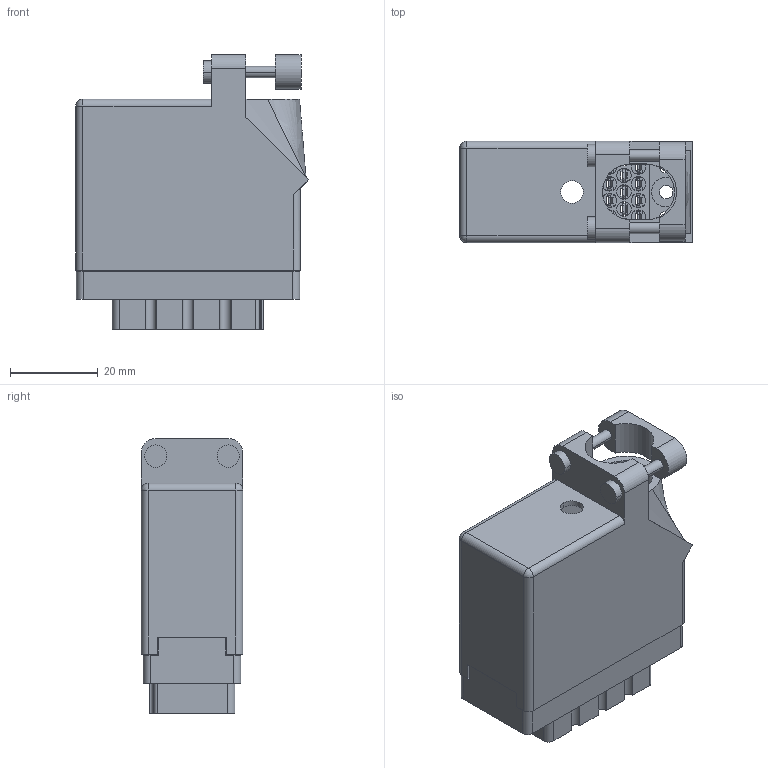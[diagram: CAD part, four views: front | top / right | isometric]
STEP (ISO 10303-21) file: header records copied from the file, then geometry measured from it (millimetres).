
FILE_DESCRIPTION (( 'STEP AP203' ), '1' );
FILE_NAME ('516-038-501-410.STEP', '2020-09-08T15:07:22', ( '' ), ( '' ), 'SwSTEP 2.0', 'SolidWorks 2020', '' );
FILE_SCHEMA (( 'CONFIG_CONTROL_DESIGN' ));
Length unit declared in the file: inch
Products named in the file (4): 516-292-001_501 Contact; 516-230-001_Plastic - 038 Top Entry; 516 Part Receptacle_038; 516-038-501-410
Assembly tree (41 placements, depth 2):
  516-038-501-410
    516 Part Receptacle_038
    516-292-001_501 Contact  x39
    516-230-001_Plastic - 038 Top Entry
Bounding box: 52.85 x 23.11 x 62.51 mm (x, y, z)
Volume: 22810.8 mm3; surface area: 35809.2 mm2
Topology: 41 solids, 41 shells, 3796 faces, 10996 edges, 7300 vertices
Faces by surface type: plane 2273, cylinder 1282, bspline 237, cone 2, sphere 2
Entity records: 37183 total; most frequent: CARTESIAN_POINT 6628, ORIENTED_EDGE 6180, DIRECTION 6050, EDGE_CURVE 3090, VECTOR 2244, LINE 2244, VERTEX_POINT 2056, AXIS2_PLACEMENT_3D 1903
